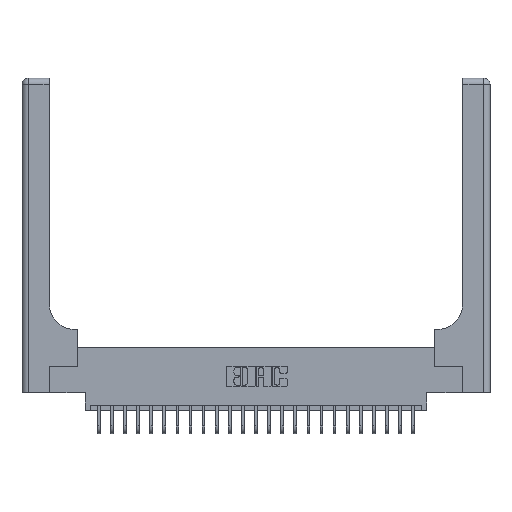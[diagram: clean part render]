
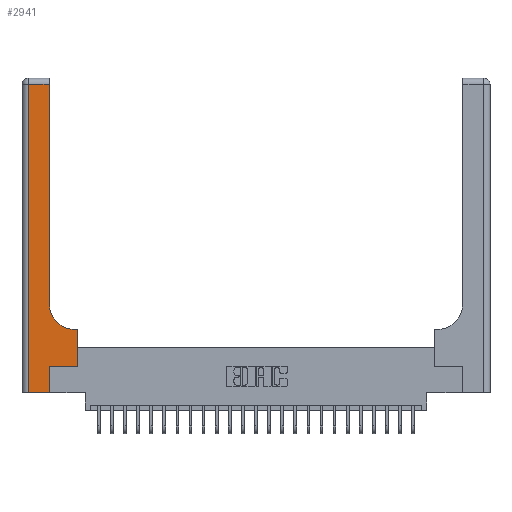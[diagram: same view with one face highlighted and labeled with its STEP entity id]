
A CAD part, top view. The second image highlights one B-rep face of the part: STEP entity #2941.
In plain terms, the highlighted planar face has unit normal (0, 0, 1).
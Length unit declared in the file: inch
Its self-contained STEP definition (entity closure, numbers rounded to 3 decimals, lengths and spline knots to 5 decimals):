
#200 = LINE ( 'NONE', #13559, #13870 ) ;
#815 = VERTEX_POINT ( 'NONE', #2265 ) ;
#1151 = EDGE_CURVE ( 'NONE', #17131, #3842, #7743, .T. ) ;
#1427 = ORIENTED_EDGE ( 'NONE', *, *, #12940, .T. ) ;
#1748 = CARTESIAN_POINT ( 'NONE',  ( 0.265, 0.25, 0.37 ) ) ;
#1995 = CARTESIAN_POINT ( 'NONE',  ( 0.265, 0., 0.37 ) ) ;
#2097 = DIRECTION ( 'NONE',  ( 0., 1., 0. ) ) ;
#2141 = VERTEX_POINT ( 'NONE', #22059 ) ;
#2233 = EDGE_CURVE ( 'NONE', #815, #13176, #8416, .T. ) ;
#2265 = CARTESIAN_POINT ( 'NONE',  ( 0.265, 0.25, 0.37 ) ) ;
#2701 = DIRECTION ( 'NONE',  ( 0., -1., 0. ) ) ;
#2757 = VERTEX_POINT ( 'NONE', #21605 ) ;
#2941 = ADVANCED_FACE ( 'NONE', ( #11466 ), #3875, .F. ) ;
#3842 = VERTEX_POINT ( 'NONE', #20595 ) ;
#3875 = PLANE ( 'NONE',  #13426 ) ;
#4304 = ORIENTED_EDGE ( 'NONE', *, *, #14291, .T. ) ;
#4401 = DIRECTION ( 'NONE',  ( 0., 1., 0. ) ) ;
#5235 = LINE ( 'NONE', #10849, #13298 ) ;
#6967 = DIRECTION ( 'NONE',  ( 1., 0., 0. ) ) ;
#7287 = EDGE_LOOP ( 'NONE', ( #8042, #21225, #19305, #1427, #20565, #12464, #4304, #24265, #12038 ) ) ;
#7743 = CIRCLE ( 'NONE', #9745, 0.25 ) ;
#8042 = ORIENTED_EDGE ( 'NONE', *, *, #16386, .T. ) ;
#8416 = LINE ( 'NONE', #1748, #25177 ) ;
#9745 = AXIS2_PLACEMENT_3D ( 'NONE', #22681, #18839, #6967 ) ;
#9865 = CARTESIAN_POINT ( 'NONE',  ( 0., 2.94, 0.37 ) ) ;
#9878 = CARTESIAN_POINT ( 'NONE',  ( 0., 3., 0.37 ) ) ;
#10849 = CARTESIAN_POINT ( 'NONE',  ( 0.06, 3., 0.37 ) ) ;
#11023 = VERTEX_POINT ( 'NONE', #24529 ) ;
#11219 = LINE ( 'NONE', #9865, #23666 ) ;
#11466 = FACE_OUTER_BOUND ( 'NONE', #7287, .T. ) ;
#11598 = VECTOR ( 'NONE', #2097, 39.37008 ) ;
#11619 = EDGE_CURVE ( 'NONE', #23374, #815, #14182, .T. ) ;
#12038 = ORIENTED_EDGE ( 'NONE', *, *, #1151, .T. ) ;
#12084 = EDGE_CURVE ( 'NONE', #2757, #17131, #200, .T. ) ;
#12464 = ORIENTED_EDGE ( 'NONE', *, *, #2233, .T. ) ;
#12581 = VERTEX_POINT ( 'NONE', #22011 ) ;
#12940 = EDGE_CURVE ( 'NONE', #2141, #23374, #19720, .T. ) ;
#13176 = VERTEX_POINT ( 'NONE', #19768 ) ;
#13249 = CARTESIAN_POINT ( 'NONE',  ( 0., 0., 0.37 ) ) ;
#13298 = VECTOR ( 'NONE', #2701, 39.37008 ) ;
#13426 = AXIS2_PLACEMENT_3D ( 'NONE', #9878, #23759, #19938 ) ;
#13429 = DIRECTION ( 'NONE',  ( 1., 0., 0. ) ) ;
#13559 = CARTESIAN_POINT ( 'NONE',  ( 0.26, 0.6, 0.37 ) ) ;
#13616 = DIRECTION ( 'NONE',  ( 0., 1., 0. ) ) ;
#13737 = LINE ( 'NONE', #25558, #11598 ) ;
#13870 = VECTOR ( 'NONE', #15464, 39.37008 ) ;
#14182 = LINE ( 'NONE', #1995, #21630 ) ;
#14291 = EDGE_CURVE ( 'NONE', #13176, #2757, #13737, .T. ) ;
#15430 = VECTOR ( 'NONE', #4401, 39.37008 ) ;
#15464 = DIRECTION ( 'NONE',  ( -1., 0., 0. ) ) ;
#15620 = DIRECTION ( 'NONE',  ( 1., 0., 0. ) ) ;
#15647 = EDGE_CURVE ( 'NONE', #12581, #2141, #5235, .T. ) ;
#15928 = DIRECTION ( 'NONE',  ( -1., 0., 0. ) ) ;
#16386 = EDGE_CURVE ( 'NONE', #3842, #11023, #17299, .T. ) ;
#17131 = VERTEX_POINT ( 'NONE', #20601 ) ;
#17299 = LINE ( 'NONE', #20213, #15430 ) ;
#18180 = VECTOR ( 'NONE', #13429, 39.37008 ) ;
#18839 = DIRECTION ( 'NONE',  ( 0., 0., -1. ) ) ;
#19305 = ORIENTED_EDGE ( 'NONE', *, *, #15647, .T. ) ;
#19639 = EDGE_CURVE ( 'NONE', #11023, #12581, #11219, .T. ) ;
#19720 = LINE ( 'NONE', #13249, #18180 ) ;
#19768 = CARTESIAN_POINT ( 'NONE',  ( 0.528, 0.25, 0.37 ) ) ;
#19938 = DIRECTION ( 'NONE',  ( -1., 0., 0. ) ) ;
#20213 = CARTESIAN_POINT ( 'NONE',  ( 0.26, 3., 0.37 ) ) ;
#20565 = ORIENTED_EDGE ( 'NONE', *, *, #11619, .T. ) ;
#20595 = CARTESIAN_POINT ( 'NONE',  ( 0.26, 0.85, 0.37 ) ) ;
#20601 = CARTESIAN_POINT ( 'NONE',  ( 0.51, 0.6, 0.37 ) ) ;
#21225 = ORIENTED_EDGE ( 'NONE', *, *, #19639, .T. ) ;
#21605 = CARTESIAN_POINT ( 'NONE',  ( 0.528, 0.6, 0.37 ) ) ;
#21630 = VECTOR ( 'NONE', #13616, 39.37008 ) ;
#22011 = CARTESIAN_POINT ( 'NONE',  ( 0.06, 2.94, 0.37 ) ) ;
#22059 = CARTESIAN_POINT ( 'NONE',  ( 0.06, 0., 0.37 ) ) ;
#22681 = CARTESIAN_POINT ( 'NONE',  ( 0.51, 0.85, 0.37 ) ) ;
#23374 = VERTEX_POINT ( 'NONE', #24578 ) ;
#23666 = VECTOR ( 'NONE', #15928, 39.37008 ) ;
#23759 = DIRECTION ( 'NONE',  ( 0., 0., -1. ) ) ;
#24265 = ORIENTED_EDGE ( 'NONE', *, *, #12084, .T. ) ;
#24529 = CARTESIAN_POINT ( 'NONE',  ( 0.26, 2.94, 0.37 ) ) ;
#24578 = CARTESIAN_POINT ( 'NONE',  ( 0.265, 0., 0.37 ) ) ;
#25177 = VECTOR ( 'NONE', #15620, 39.37008 ) ;
#25558 = CARTESIAN_POINT ( 'NONE',  ( 0.528, 0.25, 0.37 ) ) ;
